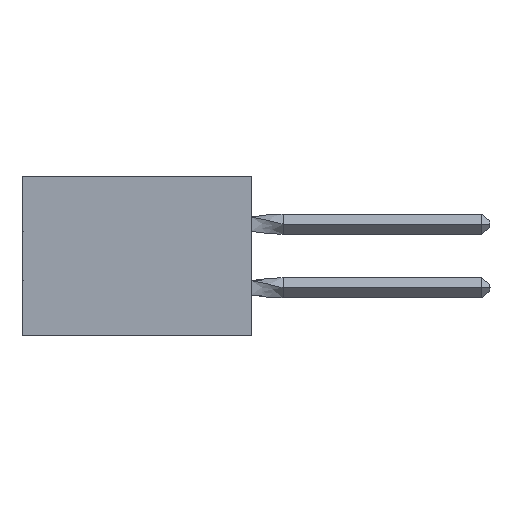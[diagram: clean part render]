
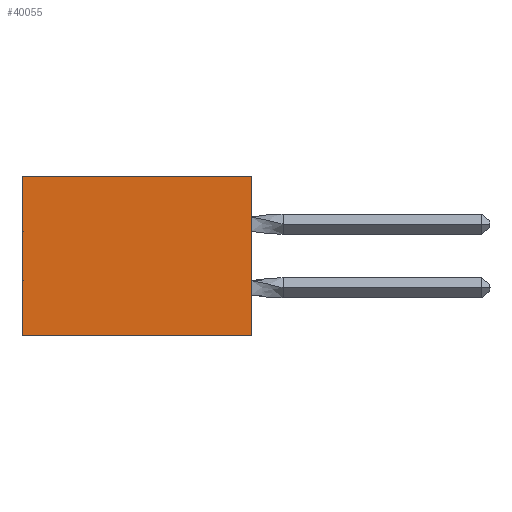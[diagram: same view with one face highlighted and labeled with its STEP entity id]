
A CAD part, left-side view. The second image highlights one B-rep face of the part: STEP entity #40055.
In plain terms, the highlighted planar face has unit normal (-1, 0, 0).
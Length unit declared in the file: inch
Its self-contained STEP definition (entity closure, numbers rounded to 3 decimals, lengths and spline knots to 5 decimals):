
#5262 = CARTESIAN_POINT ( 'NONE',  ( 0.305, 0.72, -0.5 ) ) ;
#5837 = PLANE ( 'NONE',  #26976 ) ;
#7420 = CARTESIAN_POINT ( 'NONE',  ( 0.305, 0.72, -0.5 ) ) ;
#8332 = VECTOR ( 'NONE', #8429, 39.37008 ) ;
#8429 = DIRECTION ( 'NONE',  ( 0., 1., 0. ) ) ;
#9228 = EDGE_LOOP ( 'NONE', ( #42804, #32512, #14856, #19698 ) ) ;
#13613 = VECTOR ( 'NONE', #35405, 39.37008 ) ;
#14856 = ORIENTED_EDGE ( 'NONE', *, *, #25703, .F. ) ;
#14882 = EDGE_CURVE ( 'NONE', #15142, #34250, #36914, .T. ) ;
#15142 = VERTEX_POINT ( 'NONE', #25223 ) ;
#16452 = LINE ( 'NONE', #7420, #46118 ) ;
#16529 = CARTESIAN_POINT ( 'NONE',  ( 0.305, 0.72, 0. ) ) ;
#18257 = DIRECTION ( 'NONE',  ( 0., 0., -1. ) ) ;
#19328 = FACE_OUTER_BOUND ( 'NONE', #9228, .T. ) ;
#19660 = EDGE_CURVE ( 'NONE', #39523, #39048, #38216, .T. ) ;
#19698 = ORIENTED_EDGE ( 'NONE', *, *, #19660, .T. ) ;
#24593 = DIRECTION ( 'NONE',  ( 0., 0., -1. ) ) ;
#25223 = CARTESIAN_POINT ( 'NONE',  ( 0.305, 0., -0.5 ) ) ;
#25703 = EDGE_CURVE ( 'NONE', #39523, #15142, #38813, .T. ) ;
#26976 = AXIS2_PLACEMENT_3D ( 'NONE', #31433, #35091, #42424 ) ;
#30303 = CARTESIAN_POINT ( 'NONE',  ( 0.305, 0., -0.5 ) ) ;
#30803 = VECTOR ( 'NONE', #24593, 39.37008 ) ;
#31433 = CARTESIAN_POINT ( 'NONE',  ( 0.305, 0., -0.5 ) ) ;
#32512 = ORIENTED_EDGE ( 'NONE', *, *, #14882, .F. ) ;
#34250 = VERTEX_POINT ( 'NONE', #5262 ) ;
#35091 = DIRECTION ( 'NONE',  ( 1., 0., 0. ) ) ;
#35405 = DIRECTION ( 'NONE',  ( 0., 1., 0. ) ) ;
#36914 = LINE ( 'NONE', #30303, #8332 ) ;
#38216 = LINE ( 'NONE', #42398, #13613 ) ;
#38813 = LINE ( 'NONE', #46339, #30803 ) ;
#39048 = VERTEX_POINT ( 'NONE', #16529 ) ;
#39523 = VERTEX_POINT ( 'NONE', #39922 ) ;
#39922 = CARTESIAN_POINT ( 'NONE',  ( 0.305, 0., 0. ) ) ;
#40055 = ADVANCED_FACE ( 'NONE', ( #19328 ), #5837, .F. ) ;
#42398 = CARTESIAN_POINT ( 'NONE',  ( 0.305, 0., 0. ) ) ;
#42424 = DIRECTION ( 'NONE',  ( 0., 0., -1. ) ) ;
#42804 = ORIENTED_EDGE ( 'NONE', *, *, #44014, .T. ) ;
#44014 = EDGE_CURVE ( 'NONE', #39048, #34250, #16452, .T. ) ;
#46118 = VECTOR ( 'NONE', #18257, 39.37008 ) ;
#46339 = CARTESIAN_POINT ( 'NONE',  ( 0.305, 0., -0.5 ) ) ;
